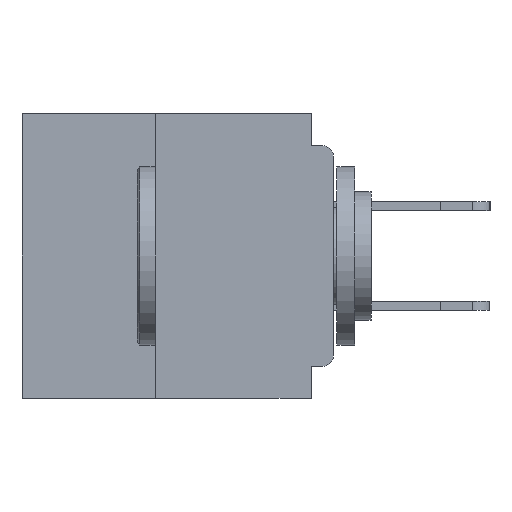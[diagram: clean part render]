
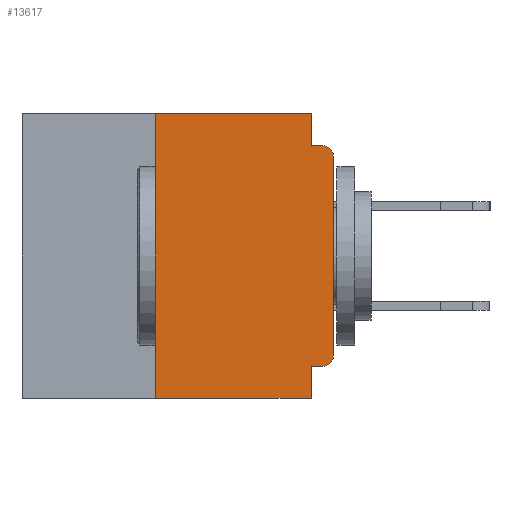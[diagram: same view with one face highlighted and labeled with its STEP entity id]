
A CAD part, left-side view. The second image highlights one B-rep face of the part: STEP entity #13617.
In plain terms, the highlighted planar face has unit normal (-1, 0, 0).
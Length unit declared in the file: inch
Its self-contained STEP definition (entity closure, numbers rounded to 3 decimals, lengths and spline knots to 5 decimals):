
#941 = ORIENTED_EDGE ( 'NONE', *, *, #16302, .F. ) ;
#1886 = EDGE_LOOP ( 'NONE', ( #27400, #18984, #941, #41447, #13955, #29120, #20701, #3796, #42030, #14563 ) ) ;
#2828 = EDGE_CURVE ( 'NONE', #33316, #6055, #7690, .T. ) ;
#2958 = CARTESIAN_POINT ( 'NONE',  ( 0., 0., 0. ) ) ;
#3092 = LINE ( 'NONE', #20783, #30668 ) ;
#3796 = ORIENTED_EDGE ( 'NONE', *, *, #15624, .F. ) ;
#4901 = DIRECTION ( 'NONE',  ( 0., 0., 1. ) ) ;
#6055 = VERTEX_POINT ( 'NONE', #35003 ) ;
#6575 = VECTOR ( 'NONE', #10891, 39.37008 ) ;
#7469 = DIRECTION ( 'NONE',  ( 0., 0., -1. ) ) ;
#7690 = LINE ( 'NONE', #12306, #6575 ) ;
#9072 = CIRCLE ( 'NONE', #40820, 0.015 ) ;
#9298 = CARTESIAN_POINT ( 'NONE',  ( 0., 0.031, -0.4 ) ) ;
#9587 = CARTESIAN_POINT ( 'NONE',  ( 0., 0.031, -0.355 ) ) ;
#9922 = VECTOR ( 'NONE', #30835, 39.37008 ) ;
#10768 = EDGE_CURVE ( 'NONE', #33834, #27089, #12031, .T. ) ;
#10891 = DIRECTION ( 'NONE',  ( 0., -1., 0. ) ) ;
#11823 = CARTESIAN_POINT ( 'NONE',  ( 0., 0.25, -0.4 ) ) ;
#11889 = AXIS2_PLACEMENT_3D ( 'NONE', #12135, #22805, #19361 ) ;
#12031 = LINE ( 'NONE', #2958, #30019 ) ;
#12069 = CARTESIAN_POINT ( 'NONE',  ( 0., 0., -0.06 ) ) ;
#12135 = CARTESIAN_POINT ( 'NONE',  ( 0., 0.437, 0. ) ) ;
#12306 = CARTESIAN_POINT ( 'NONE',  ( 0., 0.437, 0. ) ) ;
#12319 = AXIS2_PLACEMENT_3D ( 'NONE', #21135, #46182, #24758 ) ;
#12501 = VERTEX_POINT ( 'NONE', #9587 ) ;
#13174 = CARTESIAN_POINT ( 'NONE',  ( 0., 0., -0.34 ) ) ;
#13617 = ADVANCED_FACE ( 'NONE', ( #33200 ), #15794, .F. ) ;
#13955 = ORIENTED_EDGE ( 'NONE', *, *, #2828, .F. ) ;
#14563 = ORIENTED_EDGE ( 'NONE', *, *, #26070, .T. ) ;
#14934 = EDGE_CURVE ( 'NONE', #39501, #43965, #15113, .T. ) ;
#15010 = VECTOR ( 'NONE', #7469, 39.37008 ) ;
#15113 = LINE ( 'NONE', #15514, #31955 ) ;
#15289 = VERTEX_POINT ( 'NONE', #31655 ) ;
#15514 = CARTESIAN_POINT ( 'NONE',  ( 0., 0.437, -0.4 ) ) ;
#15624 = EDGE_CURVE ( 'NONE', #12501, #43965, #32440, .T. ) ;
#15794 = PLANE ( 'NONE',  #11889 ) ;
#16093 = CARTESIAN_POINT ( 'NONE',  ( 0., 0.031, -0.045 ) ) ;
#16302 = EDGE_CURVE ( 'NONE', #26546, #15289, #3092, .T. ) ;
#17513 = EDGE_CURVE ( 'NONE', #27089, #15289, #37417, .T. ) ;
#18347 = CARTESIAN_POINT ( 'NONE',  ( 0., 0., -0.355 ) ) ;
#18984 = ORIENTED_EDGE ( 'NONE', *, *, #17513, .T. ) ;
#19361 = DIRECTION ( 'NONE',  ( 0., 0., -1. ) ) ;
#20508 = CARTESIAN_POINT ( 'NONE',  ( 0., 0.015, -0.34 ) ) ;
#20701 = ORIENTED_EDGE ( 'NONE', *, *, #14934, .T. ) ;
#20783 = CARTESIAN_POINT ( 'NONE',  ( 0., 0., -0.045 ) ) ;
#20880 = DIRECTION ( 'NONE',  ( 0., 0., 1. ) ) ;
#21135 = CARTESIAN_POINT ( 'NONE',  ( 0., 0.015, -0.06 ) ) ;
#21164 = EDGE_CURVE ( 'NONE', #41729, #12501, #38194, .T. ) ;
#21771 = CARTESIAN_POINT ( 'NONE',  ( 0., 0.031, 0. ) ) ;
#22681 = EDGE_CURVE ( 'NONE', #6055, #26546, #24531, .T. ) ;
#22805 = DIRECTION ( 'NONE',  ( 1., 0., 0. ) ) ;
#23370 = EDGE_CURVE ( 'NONE', #39501, #33316, #34011, .T. ) ;
#24121 = DIRECTION ( 'NONE',  ( 0., 0., -1. ) ) ;
#24447 = VECTOR ( 'NONE', #4901, 39.37008 ) ;
#24531 = LINE ( 'NONE', #21771, #15010 ) ;
#24758 = DIRECTION ( 'NONE',  ( 0., 0., -1. ) ) ;
#26070 = EDGE_CURVE ( 'NONE', #41729, #33834, #9072, .T. ) ;
#26546 = VERTEX_POINT ( 'NONE', #16093 ) ;
#27089 = VERTEX_POINT ( 'NONE', #12069 ) ;
#27400 = ORIENTED_EDGE ( 'NONE', *, *, #10768, .T. ) ;
#28291 = CARTESIAN_POINT ( 'NONE',  ( 0., 0.25, 0. ) ) ;
#28800 = CARTESIAN_POINT ( 'NONE',  ( 0., 0.031, -0.4 ) ) ;
#29120 = ORIENTED_EDGE ( 'NONE', *, *, #23370, .F. ) ;
#30019 = VECTOR ( 'NONE', #20880, 39.37008 ) ;
#30089 = CARTESIAN_POINT ( 'NONE',  ( 0., 0.015, -0.355 ) ) ;
#30668 = VECTOR ( 'NONE', #45815, 39.37008 ) ;
#30835 = DIRECTION ( 'NONE',  ( 0., 0., -1. ) ) ;
#31655 = CARTESIAN_POINT ( 'NONE',  ( 0., 0.015, -0.045 ) ) ;
#31955 = VECTOR ( 'NONE', #44149, 39.37008 ) ;
#32440 = LINE ( 'NONE', #9298, #9922 ) ;
#33200 = FACE_OUTER_BOUND ( 'NONE', #1886, .T. ) ;
#33316 = VERTEX_POINT ( 'NONE', #28291 ) ;
#33834 = VERTEX_POINT ( 'NONE', #13174 ) ;
#34011 = LINE ( 'NONE', #11823, #24447 ) ;
#35003 = CARTESIAN_POINT ( 'NONE',  ( 0., 0.031, 0. ) ) ;
#37060 = VECTOR ( 'NONE', #43386, 39.37008 ) ;
#37417 = CIRCLE ( 'NONE', #12319, 0.015 ) ;
#38194 = LINE ( 'NONE', #18347, #37060 ) ;
#39501 = VERTEX_POINT ( 'NONE', #41879 ) ;
#40820 = AXIS2_PLACEMENT_3D ( 'NONE', #20508, #45541, #24121 ) ;
#41447 = ORIENTED_EDGE ( 'NONE', *, *, #22681, .F. ) ;
#41729 = VERTEX_POINT ( 'NONE', #30089 ) ;
#41879 = CARTESIAN_POINT ( 'NONE',  ( 0., 0.25, -0.4 ) ) ;
#42030 = ORIENTED_EDGE ( 'NONE', *, *, #21164, .F. ) ;
#43386 = DIRECTION ( 'NONE',  ( 0., 1., 0. ) ) ;
#43965 = VERTEX_POINT ( 'NONE', #28800 ) ;
#44149 = DIRECTION ( 'NONE',  ( 0., -1., 0. ) ) ;
#45541 = DIRECTION ( 'NONE',  ( -1., 0., 0. ) ) ;
#45815 = DIRECTION ( 'NONE',  ( 0., -1., 0. ) ) ;
#46182 = DIRECTION ( 'NONE',  ( -1., 0., 0. ) ) ;
